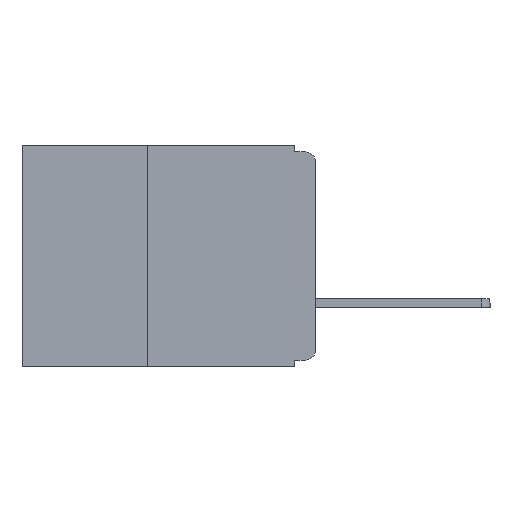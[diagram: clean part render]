
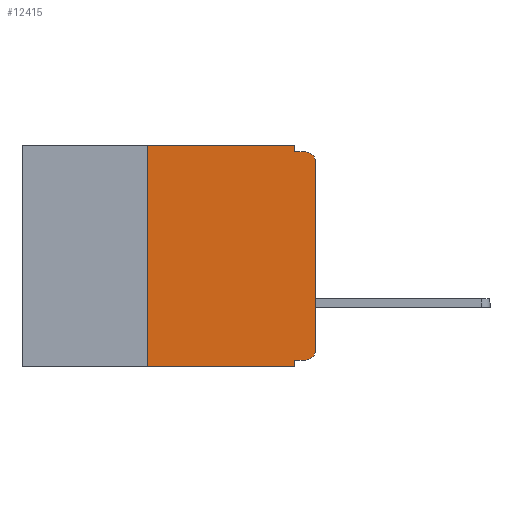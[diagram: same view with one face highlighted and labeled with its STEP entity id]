
A CAD part, left-side view. The second image highlights one B-rep face of the part: STEP entity #12415.
In plain terms, the highlighted planar face has unit normal (-1, 0, 0).
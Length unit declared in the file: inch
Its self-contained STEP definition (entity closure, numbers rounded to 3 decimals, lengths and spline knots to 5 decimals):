
#14 = CARTESIAN_POINT ( 'NONE',  ( 0., 0.015, -0.32 ) ) ;
#21 = AXIS2_PLACEMENT_3D ( 'NONE', #11482, #3212, #11529 ) ;
#618 = VERTEX_POINT ( 'NONE', #9708 ) ;
#626 = ORIENTED_EDGE ( 'NONE', *, *, #7153, .F. ) ;
#1023 = ORIENTED_EDGE ( 'NONE', *, *, #7403, .T. ) ;
#1112 = CARTESIAN_POINT ( 'NONE',  ( 0., 0., -0.025 ) ) ;
#2596 = DIRECTION ( 'NONE',  ( 0., -1., 0. ) ) ;
#2631 = CARTESIAN_POINT ( 'NONE',  ( 0., 0.25, 0. ) ) ;
#2732 = CIRCLE ( 'NONE', #12479, 0.015 ) ;
#2822 = CARTESIAN_POINT ( 'NONE',  ( 0., 0.031, -0.33 ) ) ;
#3212 = DIRECTION ( 'NONE',  ( 1., 0., 0. ) ) ;
#3485 = DIRECTION ( 'NONE',  ( 0., 0., -1. ) ) ;
#3513 = AXIS2_PLACEMENT_3D ( 'NONE', #6491, #14330, #7722 ) ;
#3557 = VERTEX_POINT ( 'NONE', #4104 ) ;
#3630 = ORIENTED_EDGE ( 'NONE', *, *, #10047, .F. ) ;
#3638 = LINE ( 'NONE', #10830, #14710 ) ;
#3696 = ORIENTED_EDGE ( 'NONE', *, *, #7330, .T. ) ;
#3769 = CARTESIAN_POINT ( 'NONE',  ( 0., 0.437, -0.33 ) ) ;
#4054 = VERTEX_POINT ( 'NONE', #14 ) ;
#4104 = CARTESIAN_POINT ( 'NONE',  ( 0., 0.031, -0.32 ) ) ;
#4389 = EDGE_LOOP ( 'NONE', ( #9400, #3696, #6153, #6524, #9706, #3630, #10076, #12959, #626, #1023 ) ) ;
#4433 = VERTEX_POINT ( 'NONE', #6705 ) ;
#4554 = CARTESIAN_POINT ( 'NONE',  ( 0., 0., 0. ) ) ;
#4752 = LINE ( 'NONE', #10909, #8020 ) ;
#4786 = LINE ( 'NONE', #7151, #5183 ) ;
#4848 = CARTESIAN_POINT ( 'NONE',  ( 0., 0.031, -0.33 ) ) ;
#5183 = VECTOR ( 'NONE', #3485, 39.37008 ) ;
#5285 = LINE ( 'NONE', #4554, #14026 ) ;
#5345 = CARTESIAN_POINT ( 'NONE',  ( 0., 0.031, -0.01 ) ) ;
#5360 = LINE ( 'NONE', #3769, #14096 ) ;
#5449 = LINE ( 'NONE', #10584, #11356 ) ;
#5547 = VECTOR ( 'NONE', #14379, 39.37008 ) ;
#6153 = ORIENTED_EDGE ( 'NONE', *, *, #6787, .F. ) ;
#6296 = CARTESIAN_POINT ( 'NONE',  ( 0., 0.015, -0.025 ) ) ;
#6491 = CARTESIAN_POINT ( 'NONE',  ( 0., 0.015, -0.305 ) ) ;
#6524 = ORIENTED_EDGE ( 'NONE', *, *, #9966, .F. ) ;
#6548 = EDGE_CURVE ( 'NONE', #13075, #10587, #5285, .T. ) ;
#6705 = CARTESIAN_POINT ( 'NONE',  ( 0., 0.031, 0. ) ) ;
#6787 = EDGE_CURVE ( 'NONE', #7460, #618, #7965, .T. ) ;
#7151 = CARTESIAN_POINT ( 'NONE',  ( 0., 0.031, 0. ) ) ;
#7153 = EDGE_CURVE ( 'NONE', #4054, #3557, #5449, .T. ) ;
#7330 = EDGE_CURVE ( 'NONE', #10587, #618, #2732, .T. ) ;
#7403 = EDGE_CURVE ( 'NONE', #4054, #13075, #11511, .T. ) ;
#7460 = VERTEX_POINT ( 'NONE', #5345 ) ;
#7488 = DIRECTION ( 'NONE',  ( 0., -1., 0. ) ) ;
#7513 = FACE_OUTER_BOUND ( 'NONE', #4389, .T. ) ;
#7523 = DIRECTION ( 'NONE',  ( 0., 0., -1. ) ) ;
#7722 = DIRECTION ( 'NONE',  ( 0., 0., -1. ) ) ;
#7965 = LINE ( 'NONE', #8742, #14176 ) ;
#8020 = VECTOR ( 'NONE', #10967, 39.37008 ) ;
#8519 = DIRECTION ( 'NONE',  ( 0., 0., 1. ) ) ;
#8742 = CARTESIAN_POINT ( 'NONE',  ( 0., 0., -0.01 ) ) ;
#8797 = LINE ( 'NONE', #2822, #5547 ) ;
#9400 = ORIENTED_EDGE ( 'NONE', *, *, #6548, .T. ) ;
#9480 = VERTEX_POINT ( 'NONE', #4848 ) ;
#9481 = CARTESIAN_POINT ( 'NONE',  ( 0., 0.25, -0.33 ) ) ;
#9483 = DIRECTION ( 'NONE',  ( 0., 1., 0. ) ) ;
#9706 = ORIENTED_EDGE ( 'NONE', *, *, #10627, .F. ) ;
#9708 = CARTESIAN_POINT ( 'NONE',  ( 0., 0.015, -0.01 ) ) ;
#9966 = EDGE_CURVE ( 'NONE', #4433, #7460, #4786, .T. ) ;
#10047 = EDGE_CURVE ( 'NONE', #10480, #10680, #3638, .T. ) ;
#10076 = ORIENTED_EDGE ( 'NONE', *, *, #10089, .T. ) ;
#10089 = EDGE_CURVE ( 'NONE', #10480, #9480, #5360, .T. ) ;
#10221 = EDGE_CURVE ( 'NONE', #3557, #9480, #8797, .T. ) ;
#10237 = CARTESIAN_POINT ( 'NONE',  ( 0., 0., -0.305 ) ) ;
#10480 = VERTEX_POINT ( 'NONE', #9481 ) ;
#10552 = DIRECTION ( 'NONE',  ( 0., 0., 1. ) ) ;
#10584 = CARTESIAN_POINT ( 'NONE',  ( 0., 0., -0.32 ) ) ;
#10587 = VERTEX_POINT ( 'NONE', #1112 ) ;
#10627 = EDGE_CURVE ( 'NONE', #10680, #4433, #4752, .T. ) ;
#10680 = VERTEX_POINT ( 'NONE', #2631 ) ;
#10830 = CARTESIAN_POINT ( 'NONE',  ( 0., 0.25, -0.33 ) ) ;
#10909 = CARTESIAN_POINT ( 'NONE',  ( 0., 0.437, 0. ) ) ;
#10967 = DIRECTION ( 'NONE',  ( 0., -1., 0. ) ) ;
#11356 = VECTOR ( 'NONE', #9483, 39.37008 ) ;
#11482 = CARTESIAN_POINT ( 'NONE',  ( 0., 0.437, 0. ) ) ;
#11511 = CIRCLE ( 'NONE', #3513, 0.015 ) ;
#11529 = DIRECTION ( 'NONE',  ( 0., 0., -1. ) ) ;
#12415 = ADVANCED_FACE ( 'NONE', ( #7513 ), #14644, .F. ) ;
#12479 = AXIS2_PLACEMENT_3D ( 'NONE', #6296, #14158, #7523 ) ;
#12959 = ORIENTED_EDGE ( 'NONE', *, *, #10221, .F. ) ;
#13075 = VERTEX_POINT ( 'NONE', #10237 ) ;
#14026 = VECTOR ( 'NONE', #10552, 39.37008 ) ;
#14096 = VECTOR ( 'NONE', #7488, 39.37008 ) ;
#14158 = DIRECTION ( 'NONE',  ( -1., 0., 0. ) ) ;
#14176 = VECTOR ( 'NONE', #2596, 39.37008 ) ;
#14330 = DIRECTION ( 'NONE',  ( -1., 0., 0. ) ) ;
#14379 = DIRECTION ( 'NONE',  ( 0., 0., -1. ) ) ;
#14644 = PLANE ( 'NONE',  #21 ) ;
#14710 = VECTOR ( 'NONE', #8519, 39.37008 ) ;
